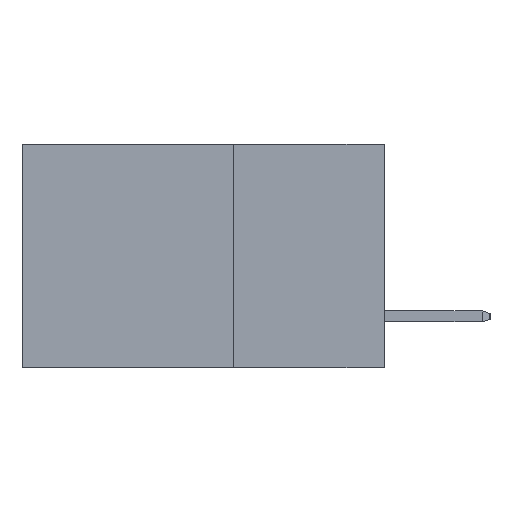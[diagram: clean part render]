
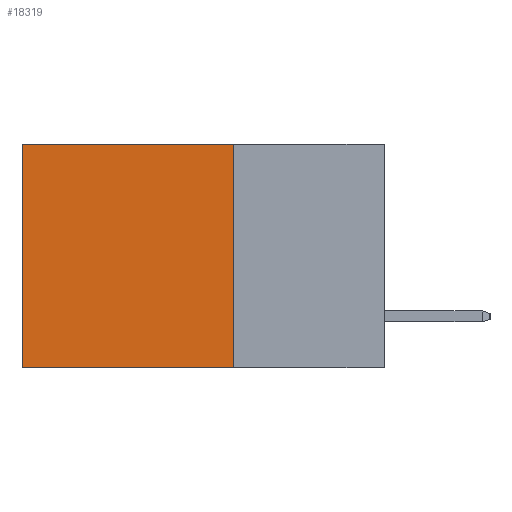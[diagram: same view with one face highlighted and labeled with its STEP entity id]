
A CAD part, left-side view. The second image highlights one B-rep face of the part: STEP entity #18319.
In plain terms, the highlighted planar face has unit normal (-1, 0, 0).
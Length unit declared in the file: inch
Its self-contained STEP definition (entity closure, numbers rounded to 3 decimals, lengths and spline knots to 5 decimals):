
#92 = CARTESIAN_POINT ( 'NONE',  ( 0.2615, 0.25, -0.37 ) ) ;
#110 = DIRECTION ( 'NONE',  ( 0., 0., -1. ) ) ;
#2609 = VECTOR ( 'NONE', #8209, 39.37008 ) ;
#2826 = CARTESIAN_POINT ( 'NONE',  ( 0.2615, 0.6, -0.37 ) ) ;
#2837 = LINE ( 'NONE', #17852, #11736 ) ;
#2924 = VERTEX_POINT ( 'NONE', #12919 ) ;
#3373 = LINE ( 'NONE', #92, #16881 ) ;
#3597 = DIRECTION ( 'NONE',  ( 0., 1., 0. ) ) ;
#4551 = CARTESIAN_POINT ( 'NONE',  ( 0.2615, 0.25, -0.37 ) ) ;
#5423 = PLANE ( 'NONE',  #21175 ) ;
#5477 = VECTOR ( 'NONE', #11506, 39.37008 ) ;
#5613 = EDGE_CURVE ( 'NONE', #14997, #20489, #10748, .T. ) ;
#7887 = CARTESIAN_POINT ( 'NONE',  ( 0.2615, 0.25, 0. ) ) ;
#8209 = DIRECTION ( 'NONE',  ( 0., 0., -1. ) ) ;
#8567 = LINE ( 'NONE', #21788, #2609 ) ;
#9925 = ORIENTED_EDGE ( 'NONE', *, *, #20501, .T. ) ;
#10203 = EDGE_LOOP ( 'NONE', ( #9925, #10550, #10886, #17281 ) ) ;
#10266 = FACE_OUTER_BOUND ( 'NONE', #10203, .T. ) ;
#10550 = ORIENTED_EDGE ( 'NONE', *, *, #21351, .F. ) ;
#10748 = LINE ( 'NONE', #11717, #5477 ) ;
#10782 = DIRECTION ( 'NONE',  ( 1., 0., 0. ) ) ;
#10886 = ORIENTED_EDGE ( 'NONE', *, *, #5613, .F. ) ;
#11030 = DIRECTION ( 'NONE',  ( 0., 1., 0. ) ) ;
#11506 = DIRECTION ( 'NONE',  ( 0., 0., -1. ) ) ;
#11717 = CARTESIAN_POINT ( 'NONE',  ( 0.2615, 0.25, -0.37 ) ) ;
#11736 = VECTOR ( 'NONE', #11030, 39.37008 ) ;
#12919 = CARTESIAN_POINT ( 'NONE',  ( 0.2615, 0.6, 0. ) ) ;
#14997 = VERTEX_POINT ( 'NONE', #7887 ) ;
#15942 = EDGE_CURVE ( 'NONE', #14997, #2924, #2837, .T. ) ;
#16881 = VECTOR ( 'NONE', #3597, 39.37008 ) ;
#17281 = ORIENTED_EDGE ( 'NONE', *, *, #15942, .T. ) ;
#17852 = CARTESIAN_POINT ( 'NONE',  ( 0.2615, 0.25, 0. ) ) ;
#18063 = VERTEX_POINT ( 'NONE', #2826 ) ;
#18319 = ADVANCED_FACE ( 'NONE', ( #10266 ), #5423, .F. ) ;
#20489 = VERTEX_POINT ( 'NONE', #4551 ) ;
#20501 = EDGE_CURVE ( 'NONE', #2924, #18063, #8567, .T. ) ;
#20948 = CARTESIAN_POINT ( 'NONE',  ( 0.2615, 0.25, -0.37 ) ) ;
#21175 = AXIS2_PLACEMENT_3D ( 'NONE', #20948, #10782, #110 ) ;
#21351 = EDGE_CURVE ( 'NONE', #20489, #18063, #3373, .T. ) ;
#21788 = CARTESIAN_POINT ( 'NONE',  ( 0.2615, 0.6, -0.37 ) ) ;
